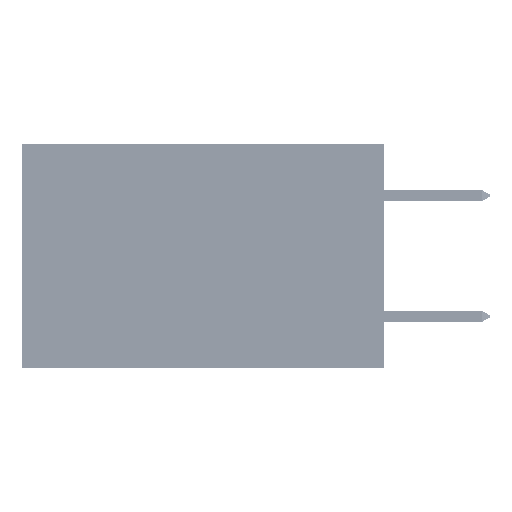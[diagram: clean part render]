
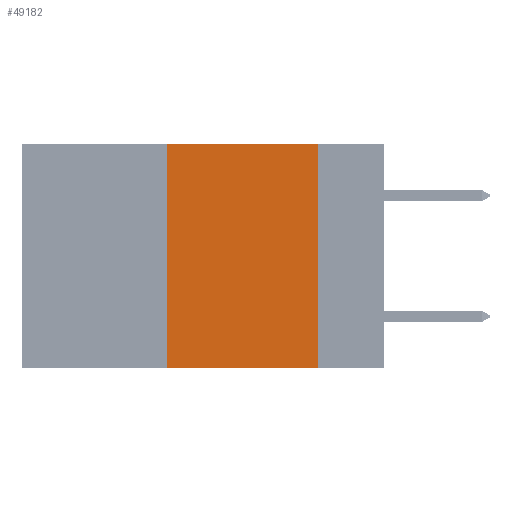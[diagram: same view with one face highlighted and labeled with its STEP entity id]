
A CAD part, left-side view. The second image highlights one B-rep face of the part: STEP entity #49182.
In plain terms, the highlighted planar face has unit normal (-1, 0, 0).
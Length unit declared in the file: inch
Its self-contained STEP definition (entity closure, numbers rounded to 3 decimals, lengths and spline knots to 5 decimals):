
#273 = ORIENTED_EDGE ( 'NONE', *, *, #45988, .F. ) ;
#1584 = EDGE_CURVE ( 'NONE', #27524, #48750, #44546, .T. ) ;
#4011 = CARTESIAN_POINT ( 'NONE',  ( 0., 0.36, -0.37 ) ) ;
#6285 = CARTESIAN_POINT ( 'NONE',  ( 0., 0.36, 0. ) ) ;
#6398 = LINE ( 'NONE', #47972, #44424 ) ;
#6774 = EDGE_LOOP ( 'NONE', ( #47262, #273, #41386, #31112 ) ) ;
#7267 = CARTESIAN_POINT ( 'NONE',  ( 0., 0.11, 0. ) ) ;
#9379 = CARTESIAN_POINT ( 'NONE',  ( 0., 0.36, 0. ) ) ;
#10302 = DIRECTION ( 'NONE',  ( 0., 0., -1. ) ) ;
#16186 = CARTESIAN_POINT ( 'NONE',  ( 0., 0.6, 0. ) ) ;
#17989 = DIRECTION ( 'NONE',  ( 0., 0., 1. ) ) ;
#18649 = FACE_OUTER_BOUND ( 'NONE', #6774, .T. ) ;
#20105 = DIRECTION ( 'NONE',  ( 1., 0., 0. ) ) ;
#20647 = DIRECTION ( 'NONE',  ( 0., -1., 0. ) ) ;
#21550 = CARTESIAN_POINT ( 'NONE',  ( 0., 0.11, -0.37 ) ) ;
#24490 = LINE ( 'NONE', #41598, #44190 ) ;
#24518 = VERTEX_POINT ( 'NONE', #9379 ) ;
#27524 = VERTEX_POINT ( 'NONE', #7267 ) ;
#29724 = DIRECTION ( 'NONE',  ( 0., -1., 0. ) ) ;
#31112 = ORIENTED_EDGE ( 'NONE', *, *, #41630, .T. ) ;
#33150 = VECTOR ( 'NONE', #17989, 39.37008 ) ;
#34034 = EDGE_CURVE ( 'NONE', #41098, #24518, #43593, .T. ) ;
#34070 = VECTOR ( 'NONE', #10302, 39.37008 ) ;
#39770 = PLANE ( 'NONE',  #50051 ) ;
#41098 = VERTEX_POINT ( 'NONE', #4011 ) ;
#41386 = ORIENTED_EDGE ( 'NONE', *, *, #34034, .F. ) ;
#41598 = CARTESIAN_POINT ( 'NONE',  ( 0., 0.6, 0. ) ) ;
#41630 = EDGE_CURVE ( 'NONE', #41098, #48750, #6398, .T. ) ;
#43593 = LINE ( 'NONE', #6285, #33150 ) ;
#44190 = VECTOR ( 'NONE', #29724, 39.37008 ) ;
#44424 = VECTOR ( 'NONE', #20647, 39.37008 ) ;
#44546 = LINE ( 'NONE', #49341, #34070 ) ;
#45988 = EDGE_CURVE ( 'NONE', #24518, #27524, #24490, .T. ) ;
#47262 = ORIENTED_EDGE ( 'NONE', *, *, #1584, .F. ) ;
#47615 = DIRECTION ( 'NONE',  ( 0., 0., -1. ) ) ;
#47972 = CARTESIAN_POINT ( 'NONE',  ( 0., 0.6, -0.37 ) ) ;
#48750 = VERTEX_POINT ( 'NONE', #21550 ) ;
#49182 = ADVANCED_FACE ( 'NONE', ( #18649 ), #39770, .F. ) ;
#49341 = CARTESIAN_POINT ( 'NONE',  ( 0., 0.11, 0. ) ) ;
#50051 = AXIS2_PLACEMENT_3D ( 'NONE', #16186, #20105, #47615 ) ;
